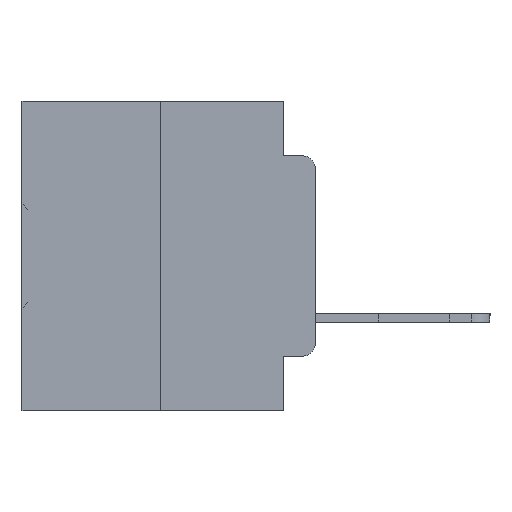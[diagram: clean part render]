
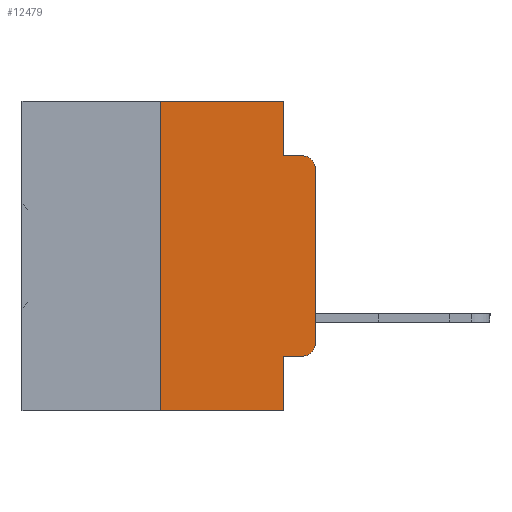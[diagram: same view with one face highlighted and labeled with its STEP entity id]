
A CAD part, left-side view. The second image highlights one B-rep face of the part: STEP entity #12479.
In plain terms, the highlighted planar face has unit normal (-1, 0, 0).
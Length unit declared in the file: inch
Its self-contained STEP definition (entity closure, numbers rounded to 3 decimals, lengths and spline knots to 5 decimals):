
#565 = VECTOR ( 'NONE', #31573, 39.37008 ) ;
#700 = VERTEX_POINT ( 'NONE', #20819 ) ;
#1261 = FACE_OUTER_BOUND ( 'NONE', #11104, .T. ) ;
#1769 = VECTOR ( 'NONE', #26294, 39.37008 ) ;
#2521 = LINE ( 'NONE', #7811, #22228 ) ;
#2763 = AXIS2_PLACEMENT_3D ( 'NONE', #25918, #9830, #28551 ) ;
#3552 = CARTESIAN_POINT ( 'NONE',  ( 0., 0.02, -0.4115 ) ) ;
#3746 = ORIENTED_EDGE ( 'NONE', *, *, #20100, .T. ) ;
#4028 = CARTESIAN_POINT ( 'NONE',  ( 0., 0.473, -0.5 ) ) ;
#4485 = VERTEX_POINT ( 'NONE', #18787 ) ;
#4750 = DIRECTION ( 'NONE',  ( 0., -1., 0. ) ) ;
#4799 = VERTEX_POINT ( 'NONE', #11492 ) ;
#4872 = CARTESIAN_POINT ( 'NONE',  ( 0., 0.473, 0. ) ) ;
#5548 = CARTESIAN_POINT ( 'NONE',  ( 0., 0.051, -0.0885 ) ) ;
#5882 = VERTEX_POINT ( 'NONE', #6286 ) ;
#5973 = CARTESIAN_POINT ( 'NONE',  ( 0., 0.051, 0. ) ) ;
#6286 = CARTESIAN_POINT ( 'NONE',  ( 0., 0., -0.3915 ) ) ;
#7811 = CARTESIAN_POINT ( 'NONE',  ( 0., 0.051, 0. ) ) ;
#7861 = LINE ( 'NONE', #20043, #13282 ) ;
#7945 = EDGE_CURVE ( 'NONE', #22311, #30927, #11409, .T. ) ;
#8020 = DIRECTION ( 'NONE',  ( 0., 0., 1. ) ) ;
#8384 = ORIENTED_EDGE ( 'NONE', *, *, #34163, .F. ) ;
#8900 = PLANE ( 'NONE',  #29743 ) ;
#9649 = ORIENTED_EDGE ( 'NONE', *, *, #31964, .F. ) ;
#9830 = DIRECTION ( 'NONE',  ( -1., 0., 0. ) ) ;
#10577 = CIRCLE ( 'NONE', #2763, 0.02 ) ;
#11104 = EDGE_LOOP ( 'NONE', ( #3746, #25580, #9649, #8384, #15160, #26052, #20657, #18151, #14543, #26091 ) ) ;
#11409 = LINE ( 'NONE', #4872, #31857 ) ;
#11492 = CARTESIAN_POINT ( 'NONE',  ( 0., 0.051, -0.5 ) ) ;
#12479 = ADVANCED_FACE ( 'NONE', ( #1261 ), #8900, .F. ) ;
#13016 = VECTOR ( 'NONE', #30297, 39.37008 ) ;
#13282 = VECTOR ( 'NONE', #17306, 39.37008 ) ;
#13795 = CIRCLE ( 'NONE', #17322, 0.02 ) ;
#13844 = LINE ( 'NONE', #16844, #13016 ) ;
#13847 = CARTESIAN_POINT ( 'NONE',  ( 0., 0.25, -0.5 ) ) ;
#13919 = LINE ( 'NONE', #15567, #565 ) ;
#14250 = DIRECTION ( 'NONE',  ( 0., 0., -1. ) ) ;
#14543 = ORIENTED_EDGE ( 'NONE', *, *, #32223, .T. ) ;
#15047 = CARTESIAN_POINT ( 'NONE',  ( 0., 0.02, -0.3915 ) ) ;
#15160 = ORIENTED_EDGE ( 'NONE', *, *, #7945, .F. ) ;
#15567 = CARTESIAN_POINT ( 'NONE',  ( 0., 0.25, 0. ) ) ;
#16844 = CARTESIAN_POINT ( 'NONE',  ( 0., 0.051, -0.4115 ) ) ;
#17306 = DIRECTION ( 'NONE',  ( 0., 0., -1. ) ) ;
#17322 = AXIS2_PLACEMENT_3D ( 'NONE', #15047, #33707, #17748 ) ;
#17748 = DIRECTION ( 'NONE',  ( 0., 0., -1. ) ) ;
#18151 = ORIENTED_EDGE ( 'NONE', *, *, #28248, .F. ) ;
#18787 = CARTESIAN_POINT ( 'NONE',  ( 0., 0.02, -0.0885 ) ) ;
#19462 = LINE ( 'NONE', #4028, #33584 ) ;
#19978 = CARTESIAN_POINT ( 'NONE',  ( 0., 0.25, 0. ) ) ;
#20043 = CARTESIAN_POINT ( 'NONE',  ( 0., 0.051, 0. ) ) ;
#20100 = EDGE_CURVE ( 'NONE', #5882, #700, #23058, .T. ) ;
#20657 = ORIENTED_EDGE ( 'NONE', *, *, #22809, .T. ) ;
#20819 = CARTESIAN_POINT ( 'NONE',  ( 0., 0., -0.1085 ) ) ;
#22092 = VERTEX_POINT ( 'NONE', #13847 ) ;
#22228 = VECTOR ( 'NONE', #23892, 39.37008 ) ;
#22311 = VERTEX_POINT ( 'NONE', #19978 ) ;
#22319 = LINE ( 'NONE', #34309, #1769 ) ;
#22809 = EDGE_CURVE ( 'NONE', #22092, #4799, #19462, .T. ) ;
#23058 = LINE ( 'NONE', #24110, #28433 ) ;
#23892 = DIRECTION ( 'NONE',  ( 0., 0., -1. ) ) ;
#24110 = CARTESIAN_POINT ( 'NONE',  ( 0., 0., 0. ) ) ;
#24328 = EDGE_CURVE ( 'NONE', #22092, #22311, #13919, .T. ) ;
#25580 = ORIENTED_EDGE ( 'NONE', *, *, #26479, .T. ) ;
#25918 = CARTESIAN_POINT ( 'NONE',  ( 0., 0.02, -0.1085 ) ) ;
#26052 = ORIENTED_EDGE ( 'NONE', *, *, #24328, .F. ) ;
#26091 = ORIENTED_EDGE ( 'NONE', *, *, #28050, .T. ) ;
#26129 = VERTEX_POINT ( 'NONE', #5548 ) ;
#26294 = DIRECTION ( 'NONE',  ( 0., -1., 0. ) ) ;
#26479 = EDGE_CURVE ( 'NONE', #700, #4485, #10577, .T. ) ;
#27634 = CARTESIAN_POINT ( 'NONE',  ( 0., 0.473, 0. ) ) ;
#28050 = EDGE_CURVE ( 'NONE', #34032, #5882, #13795, .T. ) ;
#28118 = DIRECTION ( 'NONE',  ( 0., -1., 0. ) ) ;
#28248 = EDGE_CURVE ( 'NONE', #29115, #4799, #2521, .T. ) ;
#28433 = VECTOR ( 'NONE', #8020, 39.37008 ) ;
#28551 = DIRECTION ( 'NONE',  ( 0., 0., -1. ) ) ;
#29115 = VERTEX_POINT ( 'NONE', #33304 ) ;
#29743 = AXIS2_PLACEMENT_3D ( 'NONE', #27634, #30273, #14250 ) ;
#30273 = DIRECTION ( 'NONE',  ( 1., 0., 0. ) ) ;
#30297 = DIRECTION ( 'NONE',  ( 0., -1., 0. ) ) ;
#30927 = VERTEX_POINT ( 'NONE', #5973 ) ;
#31573 = DIRECTION ( 'NONE',  ( 0., 0., 1. ) ) ;
#31857 = VECTOR ( 'NONE', #4750, 39.37008 ) ;
#31964 = EDGE_CURVE ( 'NONE', #26129, #4485, #22319, .T. ) ;
#32223 = EDGE_CURVE ( 'NONE', #29115, #34032, #13844, .T. ) ;
#33304 = CARTESIAN_POINT ( 'NONE',  ( 0., 0.051, -0.4115 ) ) ;
#33584 = VECTOR ( 'NONE', #28118, 39.37008 ) ;
#33707 = DIRECTION ( 'NONE',  ( -1., 0., 0. ) ) ;
#34032 = VERTEX_POINT ( 'NONE', #3552 ) ;
#34163 = EDGE_CURVE ( 'NONE', #30927, #26129, #7861, .T. ) ;
#34309 = CARTESIAN_POINT ( 'NONE',  ( 0., 0.051, -0.0885 ) ) ;
